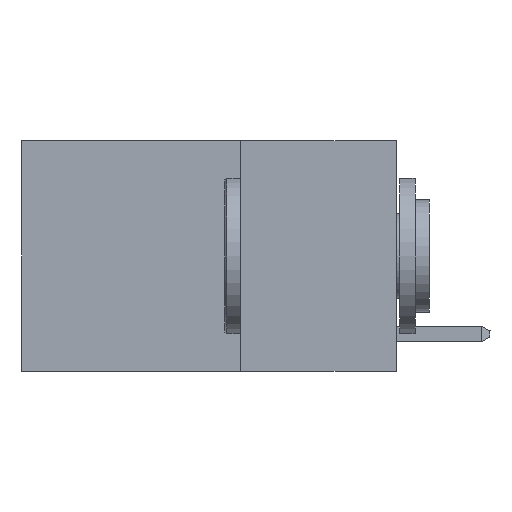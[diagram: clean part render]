
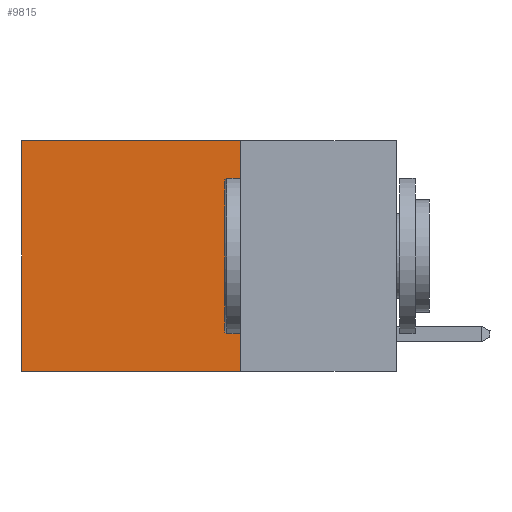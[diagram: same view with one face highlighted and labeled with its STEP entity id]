
A CAD part, left-side view. The second image highlights one B-rep face of the part: STEP entity #9815.
In plain terms, the highlighted planar face has unit normal (-1, 0, 0).
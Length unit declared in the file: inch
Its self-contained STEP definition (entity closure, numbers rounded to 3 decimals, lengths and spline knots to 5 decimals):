
#243 = CARTESIAN_POINT ( 'NONE',  ( 0.2625, 0.25, -0.37 ) ) ;
#247 = ORIENTED_EDGE ( 'NONE', *, *, #8657, .T. ) ;
#325 = VECTOR ( 'NONE', #2495, 39.37008 ) ;
#508 = ORIENTED_EDGE ( 'NONE', *, *, #9821, .T. ) ;
#1234 = DIRECTION ( 'NONE',  ( 1., 0., 0. ) ) ;
#1775 = VECTOR ( 'NONE', #13985, 39.37008 ) ;
#2326 = VECTOR ( 'NONE', #11208, 39.37008 ) ;
#2495 = DIRECTION ( 'NONE',  ( 0., 1., 0. ) ) ;
#2885 = LINE ( 'NONE', #7040, #1775 ) ;
#3730 = VECTOR ( 'NONE', #13652, 39.37008 ) ;
#3915 = VERTEX_POINT ( 'NONE', #8939 ) ;
#4355 = ORIENTED_EDGE ( 'NONE', *, *, #11900, .F. ) ;
#5617 = DIRECTION ( 'NONE',  ( 0., 0., -1. ) ) ;
#6750 = LINE ( 'NONE', #9627, #325 ) ;
#6875 = ORIENTED_EDGE ( 'NONE', *, *, #17507, .F. ) ;
#7040 = CARTESIAN_POINT ( 'NONE',  ( 0.2625, 0.6, 0. ) ) ;
#7757 = VERTEX_POINT ( 'NONE', #8386 ) ;
#8386 = CARTESIAN_POINT ( 'NONE',  ( 0.2625, 0.6, -0.37 ) ) ;
#8657 = EDGE_CURVE ( 'NONE', #3915, #9094, #12587, .T. ) ;
#8661 = EDGE_LOOP ( 'NONE', ( #508, #4355, #6875, #247 ) ) ;
#8939 = CARTESIAN_POINT ( 'NONE',  ( 0.2625, 0.25, 0. ) ) ;
#9094 = VERTEX_POINT ( 'NONE', #9803 ) ;
#9627 = CARTESIAN_POINT ( 'NONE',  ( 0.2625, 0.25, -0.37 ) ) ;
#9654 = CARTESIAN_POINT ( 'NONE',  ( 0.2625, 0.25, 0. ) ) ;
#9803 = CARTESIAN_POINT ( 'NONE',  ( 0.2625, 0.6, 0. ) ) ;
#9815 = ADVANCED_FACE ( 'NONE', ( #12772 ), #9928, .F. ) ;
#9821 = EDGE_CURVE ( 'NONE', #9094, #7757, #2885, .T. ) ;
#9928 = PLANE ( 'NONE',  #11903 ) ;
#11150 = VERTEX_POINT ( 'NONE', #243 ) ;
#11208 = DIRECTION ( 'NONE',  ( 0., 1., 0. ) ) ;
#11900 = EDGE_CURVE ( 'NONE', #11150, #7757, #6750, .T. ) ;
#11903 = AXIS2_PLACEMENT_3D ( 'NONE', #9654, #1234, #5617 ) ;
#12587 = LINE ( 'NONE', #18304, #2326 ) ;
#12772 = FACE_OUTER_BOUND ( 'NONE', #8661, .T. ) ;
#13561 = CARTESIAN_POINT ( 'NONE',  ( 0.2625, 0.25, 0. ) ) ;
#13652 = DIRECTION ( 'NONE',  ( 0., 0., -1. ) ) ;
#13985 = DIRECTION ( 'NONE',  ( 0., 0., -1. ) ) ;
#17507 = EDGE_CURVE ( 'NONE', #3915, #11150, #17697, .T. ) ;
#17697 = LINE ( 'NONE', #13561, #3730 ) ;
#18304 = CARTESIAN_POINT ( 'NONE',  ( 0.2625, 0.25, 0. ) ) ;
